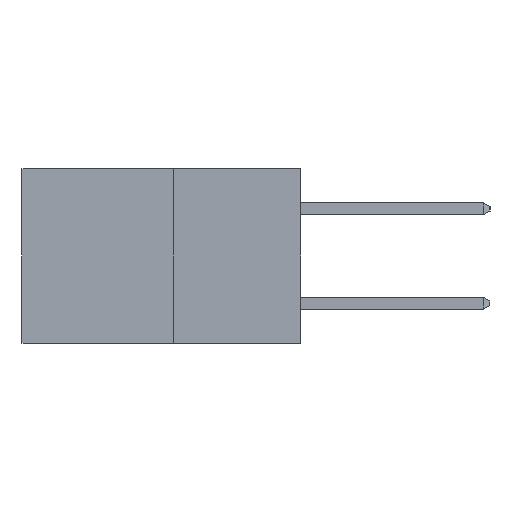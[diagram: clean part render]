
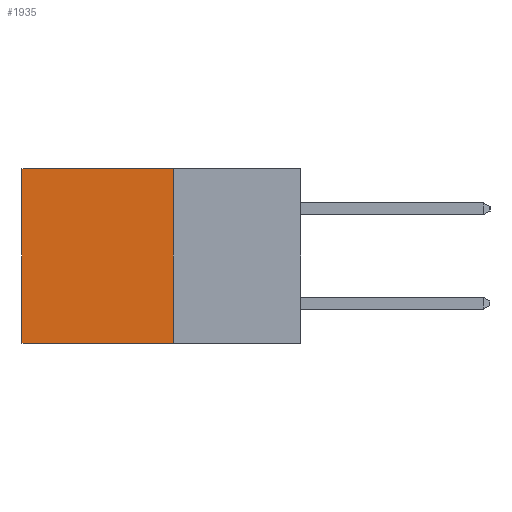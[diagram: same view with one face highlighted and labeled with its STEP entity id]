
A CAD part, left-side view. The second image highlights one B-rep face of the part: STEP entity #1935.
In plain terms, the highlighted planar face has unit normal (-1, 0, 0).
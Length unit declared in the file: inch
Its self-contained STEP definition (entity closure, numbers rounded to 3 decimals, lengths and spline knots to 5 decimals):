
#375 = CARTESIAN_POINT ( 'NONE',  ( 0.277, 0.27, -0.37 ) ) ;
#1242 = VERTEX_POINT ( 'NONE', #8614 ) ;
#1361 = VERTEX_POINT ( 'NONE', #3364 ) ;
#1394 = CARTESIAN_POINT ( 'NONE',  ( 0.277, 0.27, -0.37 ) ) ;
#1935 = ADVANCED_FACE ( 'NONE', ( #7054 ), #2645, .F. ) ;
#1962 = ORIENTED_EDGE ( 'NONE', *, *, #3000, .F. ) ;
#2639 = DIRECTION ( 'NONE',  ( 1., 0., 0. ) ) ;
#2645 = PLANE ( 'NONE',  #5847 ) ;
#3000 = EDGE_CURVE ( 'NONE', #6755, #1242, #8226, .T. ) ;
#3364 = CARTESIAN_POINT ( 'NONE',  ( 0.277, 0.27, 0. ) ) ;
#3374 = EDGE_CURVE ( 'NONE', #5628, #1242, #8414, .T. ) ;
#3713 = EDGE_LOOP ( 'NONE', ( #9153, #1962, #3769, #4155 ) ) ;
#3769 = ORIENTED_EDGE ( 'NONE', *, *, #8952, .F. ) ;
#3922 = CARTESIAN_POINT ( 'NONE',  ( 0.277, 0.27, -0.37 ) ) ;
#3930 = LINE ( 'NONE', #375, #7592 ) ;
#4155 = ORIENTED_EDGE ( 'NONE', *, *, #5833, .T. ) ;
#4693 = DIRECTION ( 'NONE',  ( 0., 1., 0. ) ) ;
#4892 = DIRECTION ( 'NONE',  ( 0., 0., -1. ) ) ;
#4921 = CARTESIAN_POINT ( 'NONE',  ( 0.277, 0.27, 0. ) ) ;
#4929 = DIRECTION ( 'NONE',  ( 0., 0., -1. ) ) ;
#5224 = VECTOR ( 'NONE', #5572, 39.37008 ) ;
#5463 = LINE ( 'NONE', #4921, #5224 ) ;
#5542 = CARTESIAN_POINT ( 'NONE',  ( 0.277, 0.59, -0.37 ) ) ;
#5572 = DIRECTION ( 'NONE',  ( 0., 1., 0. ) ) ;
#5623 = CARTESIAN_POINT ( 'NONE',  ( 0.277, 0.27, -0.37 ) ) ;
#5628 = VERTEX_POINT ( 'NONE', #8473 ) ;
#5833 = EDGE_CURVE ( 'NONE', #1361, #5628, #5463, .T. ) ;
#5847 = AXIS2_PLACEMENT_3D ( 'NONE', #1394, #2639, #4929 ) ;
#5918 = DIRECTION ( 'NONE',  ( 0., 0., -1. ) ) ;
#6309 = VECTOR ( 'NONE', #4693, 39.37008 ) ;
#6523 = VECTOR ( 'NONE', #5918, 39.37008 ) ;
#6755 = VERTEX_POINT ( 'NONE', #5623 ) ;
#7054 = FACE_OUTER_BOUND ( 'NONE', #3713, .T. ) ;
#7592 = VECTOR ( 'NONE', #4892, 39.37008 ) ;
#8226 = LINE ( 'NONE', #3922, #6309 ) ;
#8414 = LINE ( 'NONE', #5542, #6523 ) ;
#8473 = CARTESIAN_POINT ( 'NONE',  ( 0.277, 0.59, 0. ) ) ;
#8614 = CARTESIAN_POINT ( 'NONE',  ( 0.277, 0.59, -0.37 ) ) ;
#8952 = EDGE_CURVE ( 'NONE', #1361, #6755, #3930, .T. ) ;
#9153 = ORIENTED_EDGE ( 'NONE', *, *, #3374, .T. ) ;
